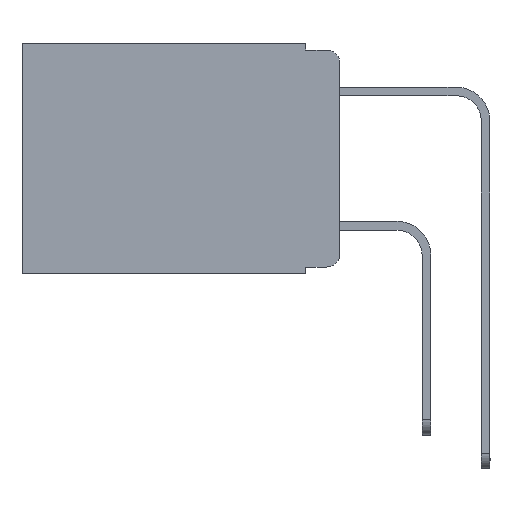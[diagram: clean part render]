
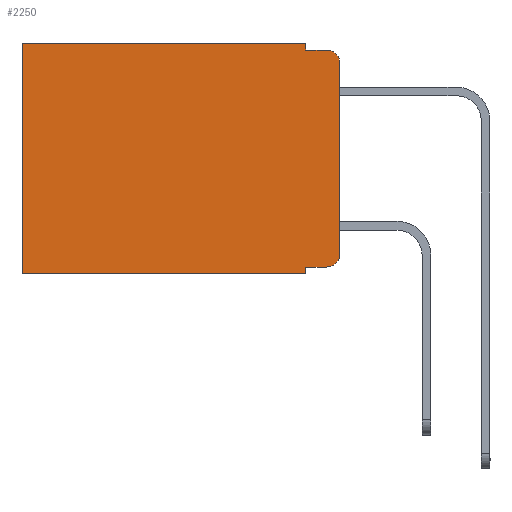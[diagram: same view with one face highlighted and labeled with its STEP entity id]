
A CAD part, left-side view. The second image highlights one B-rep face of the part: STEP entity #2250.
In plain terms, the highlighted planar face has unit normal (-1, 0, 0).
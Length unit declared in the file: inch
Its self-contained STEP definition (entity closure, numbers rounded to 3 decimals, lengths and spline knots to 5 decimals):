
#92 = VERTEX_POINT ( 'NONE', #14135 ) ;
#108 = DIRECTION ( 'NONE',  ( 0., 0., -1. ) ) ;
#752 = VECTOR ( 'NONE', #17001, 39.37008 ) ;
#1032 = VECTOR ( 'NONE', #2741, 39.37008 ) ;
#1130 = DIRECTION ( 'NONE',  ( 0., 0., -1. ) ) ;
#1357 = DIRECTION ( 'NONE',  ( 0., 0., -1. ) ) ;
#1509 = EDGE_CURVE ( 'NONE', #92, #20473, #19928, .T. ) ;
#1642 = EDGE_CURVE ( 'NONE', #20473, #8840, #2644, .T. ) ;
#1957 = EDGE_LOOP ( 'NONE', ( #14419, #6370, #7343, #20179, #2309, #6670, #4892, #4628, #16619, #2429 ) ) ;
#2081 = CARTESIAN_POINT ( 'NONE',  ( 0.298, 0.473, 0. ) ) ;
#2250 = ADVANCED_FACE ( 'NONE', ( #6435 ), #13030, .F. ) ;
#2309 = ORIENTED_EDGE ( 'NONE', *, *, #7789, .T. ) ;
#2429 = ORIENTED_EDGE ( 'NONE', *, *, #11340, .T. ) ;
#2601 = EDGE_CURVE ( 'NONE', #13543, #19887, #5988, .T. ) ;
#2644 = LINE ( 'NONE', #2953, #10768 ) ;
#2741 = DIRECTION ( 'NONE',  ( 0., 0., -1. ) ) ;
#2886 = VERTEX_POINT ( 'NONE', #6729 ) ;
#2953 = CARTESIAN_POINT ( 'NONE',  ( 0.298, 0., -0.343 ) ) ;
#4599 = CARTESIAN_POINT ( 'NONE',  ( 0.298, 0.02, -0.333 ) ) ;
#4628 = ORIENTED_EDGE ( 'NONE', *, *, #1509, .F. ) ;
#4892 = ORIENTED_EDGE ( 'NONE', *, *, #1642, .F. ) ;
#5330 = LINE ( 'NONE', #10019, #7475 ) ;
#5988 = LINE ( 'NONE', #8974, #7757 ) ;
#6184 = VECTOR ( 'NONE', #12846, 39.37008 ) ;
#6364 = CARTESIAN_POINT ( 'NONE',  ( 0.298, 0.051, -0.333 ) ) ;
#6370 = ORIENTED_EDGE ( 'NONE', *, *, #17152, .T. ) ;
#6435 = FACE_OUTER_BOUND ( 'NONE', #1957, .T. ) ;
#6653 = DIRECTION ( 'NONE',  ( 1., 0., 0. ) ) ;
#6670 = ORIENTED_EDGE ( 'NONE', *, *, #12392, .T. ) ;
#6729 = CARTESIAN_POINT ( 'NONE',  ( 0.298, 0.051, 0. ) ) ;
#7343 = ORIENTED_EDGE ( 'NONE', *, *, #16203, .F. ) ;
#7475 = VECTOR ( 'NONE', #18072, 39.37008 ) ;
#7733 = VECTOR ( 'NONE', #18538, 39.37008 ) ;
#7757 = VECTOR ( 'NONE', #1130, 39.37008 ) ;
#7789 = EDGE_CURVE ( 'NONE', #2886, #19315, #17102, .T. ) ;
#8179 = LINE ( 'NONE', #6364, #6184 ) ;
#8613 = CARTESIAN_POINT ( 'NONE',  ( 0.298, 0.051, 0. ) ) ;
#8840 = VERTEX_POINT ( 'NONE', #12808 ) ;
#8974 = CARTESIAN_POINT ( 'NONE',  ( 0.298, 0., 0. ) ) ;
#10019 = CARTESIAN_POINT ( 'NONE',  ( 0.298, 0.051, -0.01 ) ) ;
#10768 = VECTOR ( 'NONE', #12313, 39.37008 ) ;
#10902 = AXIS2_PLACEMENT_3D ( 'NONE', #14394, #20840, #1357 ) ;
#11108 = CARTESIAN_POINT ( 'NONE',  ( 0.298, 0., 0. ) ) ;
#11278 = VECTOR ( 'NONE', #108, 39.37008 ) ;
#11340 = EDGE_CURVE ( 'NONE', #20823, #19887, #12580, .T. ) ;
#12313 = DIRECTION ( 'NONE',  ( 0., 1., 0. ) ) ;
#12392 = EDGE_CURVE ( 'NONE', #19315, #8840, #14191, .T. ) ;
#12580 = CIRCLE ( 'NONE', #12939, 0.02 ) ;
#12621 = LINE ( 'NONE', #14619, #11278 ) ;
#12808 = CARTESIAN_POINT ( 'NONE',  ( 0.298, 0.473, -0.343 ) ) ;
#12846 = DIRECTION ( 'NONE',  ( 0., -1., 0. ) ) ;
#12939 = AXIS2_PLACEMENT_3D ( 'NONE', #15312, #15199, #16798 ) ;
#13030 = PLANE ( 'NONE',  #15879 ) ;
#13227 = DIRECTION ( 'NONE',  ( 0., 0., -1. ) ) ;
#13261 = CARTESIAN_POINT ( 'NONE',  ( 0.298, 0.051, -0.01 ) ) ;
#13543 = VERTEX_POINT ( 'NONE', #16570 ) ;
#14135 = CARTESIAN_POINT ( 'NONE',  ( 0.298, 0.051, -0.333 ) ) ;
#14191 = LINE ( 'NONE', #17262, #1032 ) ;
#14394 = CARTESIAN_POINT ( 'NONE',  ( 0.298, 0.02, -0.03 ) ) ;
#14419 = ORIENTED_EDGE ( 'NONE', *, *, #2601, .F. ) ;
#14619 = CARTESIAN_POINT ( 'NONE',  ( 0.298, 0.051, 0. ) ) ;
#14966 = CIRCLE ( 'NONE', #10902, 0.02 ) ;
#15199 = DIRECTION ( 'NONE',  ( -1., 0., 0. ) ) ;
#15312 = CARTESIAN_POINT ( 'NONE',  ( 0.298, 0.02, -0.313 ) ) ;
#15756 = VERTEX_POINT ( 'NONE', #13261 ) ;
#15879 = AXIS2_PLACEMENT_3D ( 'NONE', #11108, #6653, #13227 ) ;
#16203 = EDGE_CURVE ( 'NONE', #15756, #18244, #5330, .T. ) ;
#16337 = CARTESIAN_POINT ( 'NONE',  ( 0.298, 0.02, -0.01 ) ) ;
#16570 = CARTESIAN_POINT ( 'NONE',  ( 0.298, 0., -0.03 ) ) ;
#16619 = ORIENTED_EDGE ( 'NONE', *, *, #18236, .T. ) ;
#16798 = DIRECTION ( 'NONE',  ( 0., 0., -1. ) ) ;
#17001 = DIRECTION ( 'NONE',  ( 0., 1., 0. ) ) ;
#17102 = LINE ( 'NONE', #18565, #752 ) ;
#17152 = EDGE_CURVE ( 'NONE', #13543, #18244, #14966, .T. ) ;
#17262 = CARTESIAN_POINT ( 'NONE',  ( 0.298, 0.473, 0. ) ) ;
#17558 = CARTESIAN_POINT ( 'NONE',  ( 0.298, 0.051, -0.343 ) ) ;
#18072 = DIRECTION ( 'NONE',  ( 0., -1., 0. ) ) ;
#18236 = EDGE_CURVE ( 'NONE', #92, #20823, #8179, .T. ) ;
#18244 = VERTEX_POINT ( 'NONE', #16337 ) ;
#18538 = DIRECTION ( 'NONE',  ( 0., 0., -1. ) ) ;
#18565 = CARTESIAN_POINT ( 'NONE',  ( 0.298, 0., 0. ) ) ;
#18648 = CARTESIAN_POINT ( 'NONE',  ( 0.298, 0., -0.313 ) ) ;
#18684 = EDGE_CURVE ( 'NONE', #2886, #15756, #12621, .T. ) ;
#19315 = VERTEX_POINT ( 'NONE', #2081 ) ;
#19887 = VERTEX_POINT ( 'NONE', #18648 ) ;
#19928 = LINE ( 'NONE', #8613, #7733 ) ;
#20179 = ORIENTED_EDGE ( 'NONE', *, *, #18684, .F. ) ;
#20473 = VERTEX_POINT ( 'NONE', #17558 ) ;
#20823 = VERTEX_POINT ( 'NONE', #4599 ) ;
#20840 = DIRECTION ( 'NONE',  ( -1., 0., 0. ) ) ;
